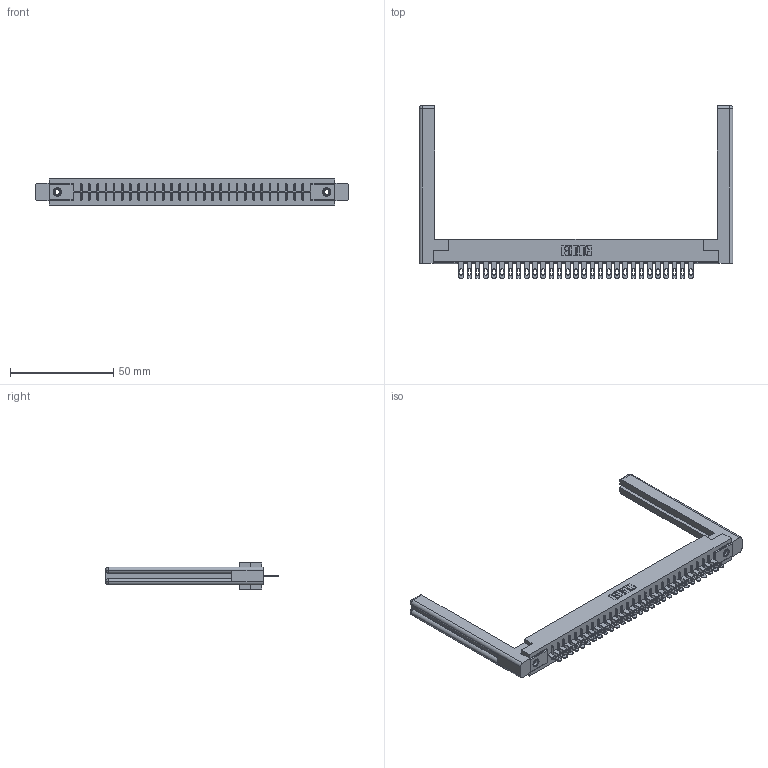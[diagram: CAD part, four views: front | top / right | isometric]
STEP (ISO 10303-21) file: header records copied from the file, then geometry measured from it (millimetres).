
FILE_DESCRIPTION (( 'STEP AP203' ), '1' );
FILE_NAME ('316-029-400-158.STEP', '2020-09-22T23:52:53', ( '' ), ( '' ), 'SwSTEP 2.0', 'SolidWorks 2020', '' );
FILE_SCHEMA (( 'CONFIG_CONTROL_DESIGN' ));
Length unit declared in the file: inch
Products named in the file (5): 316-029-400-158; 306-290-001_100; 306 Part_.156 Dia; 345-250-001_345-250-001-102; 307-220-058
Assembly tree (34 placements, depth 2):
  316-029-400-158
    306 Part_.156 Dia
    306-290-001_100  x29
    345-250-001_345-250-001-102  x2
    307-220-058  x2
Bounding box: 151.54 x 83.52 x 12.7 mm (x, y, z)
Volume: 23809.2 mm3; surface area: 22662.8 mm2
Topology: 34 solids, 34 shells, 2462 faces, 6905 edges, 4434 vertices
Faces by surface type: plane 1602, cylinder 720, sphere 116, cone 12, torus 12
Entity records: 31525 total; most frequent: CARTESIAN_POINT 5301, ORIENTED_EDGE 5196, DIRECTION 5184, EDGE_CURVE 2598, VECTOR 2018, LINE 2018, VERTEX_POINT 1646, AXIS2_PLACEMENT_3D 1583
